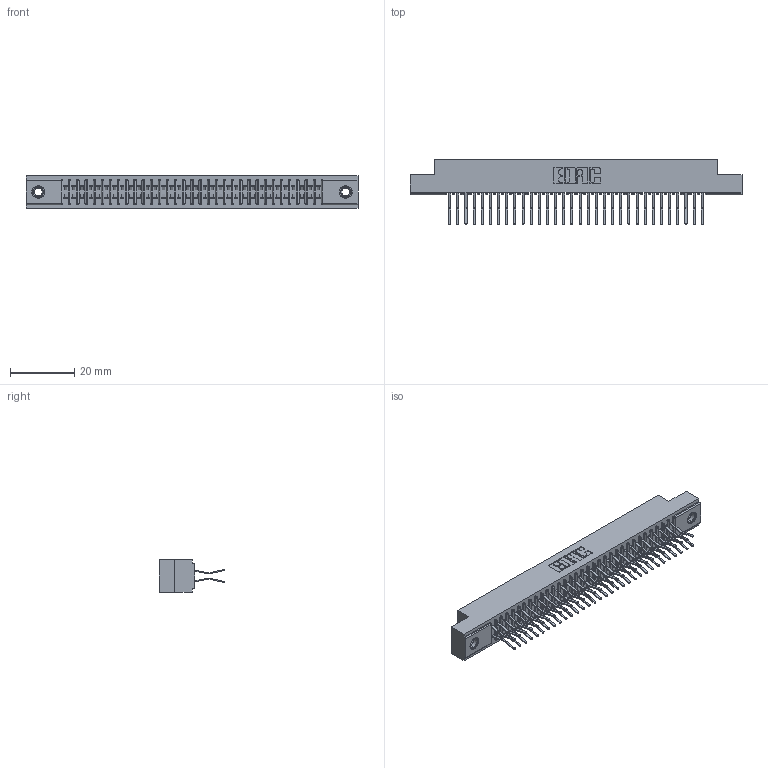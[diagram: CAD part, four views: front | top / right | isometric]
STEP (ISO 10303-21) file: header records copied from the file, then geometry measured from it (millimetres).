
FILE_DESCRIPTION (( 'STEP AP203' ), '1' );
FILE_NAME ('391-064-560-207.STEP', '2018-08-09T13:21:59', ( '' ), ( '' ), 'SwSTEP 2.0', 'SolidWorks 2016', '' );
FILE_SCHEMA (( 'CONFIG_CONTROL_DESIGN' ));
Length unit declared in the file: inch
Products named in the file (4): 341-292-001_341-292-160; 345-250-001_345-250-005-103; 391-064-560-207; 341 Part_.156 (3.96) Dia Mounting Holes
Assembly tree (67 placements, depth 2):
  391-064-560-207
    341 Part_.156 (3.96) Dia Mounting Holes
    341-292-001_341-292-160  x64
    345-250-001_345-250-005-103  x2
Bounding box: 103.5 x 20.37 x 10.16 mm (x, y, z)
Volume: 7684.5 mm3; surface area: 13834.3 mm2
Topology: 67 solids, 67 shells, 4656 faces, 13476 edges, 8738 vertices
Faces by surface type: plane 2660, cylinder 1852, sphere 66, torus 66, cone 12
Entity records: 41384 total; most frequent: CARTESIAN_POINT 6863, ORIENTED_EDGE 6812, DIRECTION 6682, EDGE_CURVE 3406, LINE 2732, VECTOR 2732, VERTEX_POINT 2156, AXIS2_PLACEMENT_3D 1975
